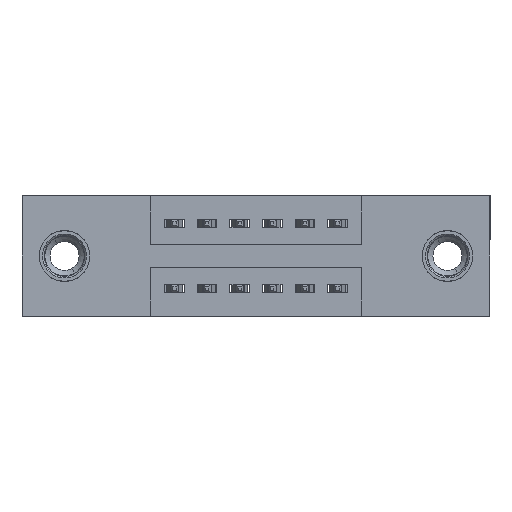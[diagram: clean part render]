
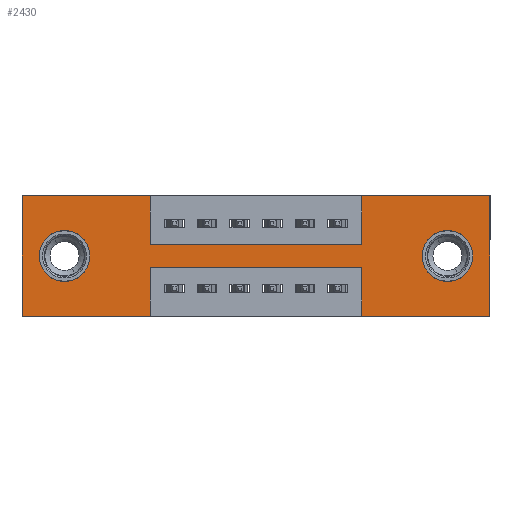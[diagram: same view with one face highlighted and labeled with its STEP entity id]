
A CAD part, front view. The second image highlights one B-rep face of the part: STEP entity #2430.
In plain terms, the highlighted planar face has unit normal (0, -1, 0).
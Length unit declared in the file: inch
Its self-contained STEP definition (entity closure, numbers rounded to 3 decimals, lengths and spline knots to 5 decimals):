
#135 = VECTOR ( 'NONE', #530, 39.37008 ) ;
#219 = CARTESIAN_POINT ( 'NONE',  ( 1.0425, 0., -0.37 ) ) ;
#243 = VERTEX_POINT ( 'NONE', #446 ) ;
#343 = CARTESIAN_POINT ( 'NONE',  ( 0., 0., -0.37 ) ) ;
#446 = CARTESIAN_POINT ( 'NONE',  ( 1.435, 0., -0.37 ) ) ;
#457 = AXIS2_PLACEMENT_3D ( 'NONE', #11871, #5175, #12933 ) ;
#530 = DIRECTION ( 'NONE',  ( 0., 0., -1. ) ) ;
#587 = EDGE_CURVE ( 'NONE', #9913, #12338, #13255, .T. ) ;
#811 = EDGE_CURVE ( 'NONE', #7252, #1962, #5625, .T. ) ;
#879 = CIRCLE ( 'NONE', #991, 0.078 ) ;
#899 = ORIENTED_EDGE ( 'NONE', *, *, #9213, .F. ) ;
#991 = AXIS2_PLACEMENT_3D ( 'NONE', #6769, #6752, #6735 ) ;
#1046 = DIRECTION ( 'NONE',  ( 0., 1., 0. ) ) ;
#1078 = CARTESIAN_POINT ( 'NONE',  ( 1.305, 0., -0.185 ) ) ;
#1255 = EDGE_CURVE ( 'NONE', #6363, #8230, #2990, .T. ) ;
#1276 = VERTEX_POINT ( 'NONE', #3013 ) ;
#1614 = ORIENTED_EDGE ( 'NONE', *, *, #587, .F. ) ;
#1720 = CIRCLE ( 'NONE', #8643, 0.078 ) ;
#1917 = EDGE_CURVE ( 'NONE', #8348, #11633, #879, .T. ) ;
#1962 = VERTEX_POINT ( 'NONE', #4195 ) ;
#2200 = DIRECTION ( 'NONE',  ( 0., 0., -1. ) ) ;
#2403 = CIRCLE ( 'NONE', #13625, 0.078 ) ;
#2430 = ADVANCED_FACE ( 'NONE', ( #9476, #6102, #3129 ), #8458, .T. ) ;
#2528 = DIRECTION ( 'NONE',  ( 0., 0., -1. ) ) ;
#2545 = CARTESIAN_POINT ( 'NONE',  ( 0.3925, 0., -0.37 ) ) ;
#2904 = DIRECTION ( 'NONE',  ( -1., 0., 0. ) ) ;
#2976 = ORIENTED_EDGE ( 'NONE', *, *, #5155, .T. ) ;
#2990 = LINE ( 'NONE', #3721, #5611 ) ;
#3013 = CARTESIAN_POINT ( 'NONE',  ( 0.13, 0., -0.263 ) ) ;
#3057 = VECTOR ( 'NONE', #3636, 39.37008 ) ;
#3074 = CARTESIAN_POINT ( 'NONE',  ( 0.3925, 0., -0.22 ) ) ;
#3129 = FACE_OUTER_BOUND ( 'NONE', #7945, .T. ) ;
#3355 = CARTESIAN_POINT ( 'NONE',  ( 1.0425, 0., -0.15 ) ) ;
#3531 = DIRECTION ( 'NONE',  ( 1., 0., 0. ) ) ;
#3549 = EDGE_CURVE ( 'NONE', #8230, #6607, #10190, .T. ) ;
#3564 = EDGE_LOOP ( 'NONE', ( #2976, #11907 ) ) ;
#3636 = DIRECTION ( 'NONE',  ( 0., 0., -1. ) ) ;
#3654 = DIRECTION ( 'NONE',  ( 1., 0., 0. ) ) ;
#3661 = ORIENTED_EDGE ( 'NONE', *, *, #14028, .F. ) ;
#3677 = DIRECTION ( 'NONE',  ( -1., 0., 0. ) ) ;
#3721 = CARTESIAN_POINT ( 'NONE',  ( 0.3925, 0., -0.22 ) ) ;
#4195 = CARTESIAN_POINT ( 'NONE',  ( 1.0425, 0., 0. ) ) ;
#4563 = CARTESIAN_POINT ( 'NONE',  ( 0.3925, 0., 0. ) ) ;
#4630 = VECTOR ( 'NONE', #3531, 39.37008 ) ;
#4744 = EDGE_CURVE ( 'NONE', #1276, #12189, #2403, .T. ) ;
#4755 = CARTESIAN_POINT ( 'NONE',  ( 1.0425, 0., -0.37 ) ) ;
#4912 = LINE ( 'NONE', #10435, #13706 ) ;
#5014 = CARTESIAN_POINT ( 'NONE',  ( 1.435, 0., 0. ) ) ;
#5155 = EDGE_CURVE ( 'NONE', #12189, #1276, #9013, .T. ) ;
#5175 = DIRECTION ( 'NONE',  ( 0., 1., 0. ) ) ;
#5250 = ORIENTED_EDGE ( 'NONE', *, *, #8855, .T. ) ;
#5261 = EDGE_LOOP ( 'NONE', ( #5250, #14034 ) ) ;
#5561 = EDGE_CURVE ( 'NONE', #243, #9596, #12590, .T. ) ;
#5611 = VECTOR ( 'NONE', #2904, 39.37008 ) ;
#5625 = LINE ( 'NONE', #10940, #7953 ) ;
#5860 = DIRECTION ( 'NONE',  ( 0., 0., 1. ) ) ;
#6029 = LINE ( 'NONE', #7006, #3057 ) ;
#6042 = VECTOR ( 'NONE', #8165, 39.37008 ) ;
#6102 = FACE_BOUND ( 'NONE', #3564, .T. ) ;
#6363 = VERTEX_POINT ( 'NONE', #10796 ) ;
#6518 = CARTESIAN_POINT ( 'NONE',  ( 0.13, 0., -0.107 ) ) ;
#6558 = CARTESIAN_POINT ( 'NONE',  ( 1.305, 0., -0.263 ) ) ;
#6607 = VERTEX_POINT ( 'NONE', #8963 ) ;
#6735 = DIRECTION ( 'NONE',  ( 0., 0., -1. ) ) ;
#6752 = DIRECTION ( 'NONE',  ( 0., 1., 0. ) ) ;
#6769 = CARTESIAN_POINT ( 'NONE',  ( 1.305, 0., -0.185 ) ) ;
#6955 = VERTEX_POINT ( 'NONE', #11870 ) ;
#7006 = CARTESIAN_POINT ( 'NONE',  ( 1.435, 0., 0. ) ) ;
#7252 = VERTEX_POINT ( 'NONE', #3355 ) ;
#7458 = CARTESIAN_POINT ( 'NONE',  ( 0., 0., 0. ) ) ;
#7752 = ORIENTED_EDGE ( 'NONE', *, *, #10187, .F. ) ;
#7776 = CARTESIAN_POINT ( 'NONE',  ( 0.13, 0., -0.185 ) ) ;
#7945 = EDGE_LOOP ( 'NONE', ( #9326, #12249, #3661, #12889, #7752, #13873, #11400, #9169, #899, #1614, #8289, #11576 ) ) ;
#7953 = VECTOR ( 'NONE', #9602, 39.37008 ) ;
#8165 = DIRECTION ( 'NONE',  ( 0., 0., 1. ) ) ;
#8230 = VERTEX_POINT ( 'NONE', #3074 ) ;
#8269 = DIRECTION ( 'NONE',  ( 0., 0., -1. ) ) ;
#8289 = ORIENTED_EDGE ( 'NONE', *, *, #9682, .F. ) ;
#8337 = EDGE_CURVE ( 'NONE', #6607, #6955, #12849, .T. ) ;
#8348 = VERTEX_POINT ( 'NONE', #6558 ) ;
#8370 = DIRECTION ( 'NONE',  ( 0., -1., 0. ) ) ;
#8407 = CARTESIAN_POINT ( 'NONE',  ( 0.3925, 0., -0.15 ) ) ;
#8458 = PLANE ( 'NONE',  #11943 ) ;
#8643 = AXIS2_PLACEMENT_3D ( 'NONE', #1078, #8946, #2200 ) ;
#8773 = CARTESIAN_POINT ( 'NONE',  ( 0., 0., -0.37 ) ) ;
#8855 = EDGE_CURVE ( 'NONE', #11633, #8348, #1720, .T. ) ;
#8915 = DIRECTION ( 'NONE',  ( 0., 0., 1. ) ) ;
#8946 = DIRECTION ( 'NONE',  ( 0., 1., 0. ) ) ;
#8963 = CARTESIAN_POINT ( 'NONE',  ( 0.3925, 0., -0.37 ) ) ;
#9013 = CIRCLE ( 'NONE', #457, 0.078 ) ;
#9169 = ORIENTED_EDGE ( 'NONE', *, *, #10774, .F. ) ;
#9213 = EDGE_CURVE ( 'NONE', #12338, #12538, #12013, .T. ) ;
#9321 = DIRECTION ( 'NONE',  ( 1., 0., 0. ) ) ;
#9326 = ORIENTED_EDGE ( 'NONE', *, *, #3549, .F. ) ;
#9476 = FACE_BOUND ( 'NONE', #5261, .T. ) ;
#9596 = VERTEX_POINT ( 'NONE', #219 ) ;
#9602 = DIRECTION ( 'NONE',  ( 0., 0., 1. ) ) ;
#9682 = EDGE_CURVE ( 'NONE', #6955, #9913, #12003, .T. ) ;
#9692 = VECTOR ( 'NONE', #3677, 39.37008 ) ;
#9828 = VECTOR ( 'NONE', #2528, 39.37008 ) ;
#9913 = VERTEX_POINT ( 'NONE', #7458 ) ;
#9935 = CARTESIAN_POINT ( 'NONE',  ( 0., 0., -0.37 ) ) ;
#9999 = VECTOR ( 'NONE', #13167, 39.37008 ) ;
#10187 = EDGE_CURVE ( 'NONE', #13062, #243, #6029, .T. ) ;
#10190 = LINE ( 'NONE', #2545, #9828 ) ;
#10418 = VECTOR ( 'NONE', #9321, 39.37008 ) ;
#10435 = CARTESIAN_POINT ( 'NONE',  ( 0., 0., 0. ) ) ;
#10616 = LINE ( 'NONE', #11339, #4630 ) ;
#10774 = EDGE_CURVE ( 'NONE', #12538, #7252, #10616, .T. ) ;
#10796 = CARTESIAN_POINT ( 'NONE',  ( 1.0425, 0., -0.22 ) ) ;
#10940 = CARTESIAN_POINT ( 'NONE',  ( 1.0425, 0., 0. ) ) ;
#11339 = CARTESIAN_POINT ( 'NONE',  ( 0.3925, 0., -0.15 ) ) ;
#11400 = ORIENTED_EDGE ( 'NONE', *, *, #811, .F. ) ;
#11567 = VECTOR ( 'NONE', #5860, 39.37008 ) ;
#11576 = ORIENTED_EDGE ( 'NONE', *, *, #8337, .F. ) ;
#11633 = VERTEX_POINT ( 'NONE', #14129 ) ;
#11870 = CARTESIAN_POINT ( 'NONE',  ( 0., 0., -0.37 ) ) ;
#11871 = CARTESIAN_POINT ( 'NONE',  ( 0.13, 0., -0.185 ) ) ;
#11891 = CARTESIAN_POINT ( 'NONE',  ( 0., 0., 0. ) ) ;
#11907 = ORIENTED_EDGE ( 'NONE', *, *, #4744, .T. ) ;
#11943 = AXIS2_PLACEMENT_3D ( 'NONE', #8773, #8370, #8269 ) ;
#12003 = LINE ( 'NONE', #13629, #6042 ) ;
#12013 = LINE ( 'NONE', #13783, #135 ) ;
#12189 = VERTEX_POINT ( 'NONE', #6518 ) ;
#12249 = ORIENTED_EDGE ( 'NONE', *, *, #1255, .F. ) ;
#12338 = VERTEX_POINT ( 'NONE', #4563 ) ;
#12538 = VERTEX_POINT ( 'NONE', #8407 ) ;
#12590 = LINE ( 'NONE', #343, #9692 ) ;
#12849 = LINE ( 'NONE', #9935, #9999 ) ;
#12889 = ORIENTED_EDGE ( 'NONE', *, *, #5561, .F. ) ;
#12933 = DIRECTION ( 'NONE',  ( 0., 0., 1. ) ) ;
#13062 = VERTEX_POINT ( 'NONE', #5014 ) ;
#13167 = DIRECTION ( 'NONE',  ( -1., 0., 0. ) ) ;
#13255 = LINE ( 'NONE', #11891, #10418 ) ;
#13625 = AXIS2_PLACEMENT_3D ( 'NONE', #7776, #1046, #8915 ) ;
#13629 = CARTESIAN_POINT ( 'NONE',  ( 0., 0., 0. ) ) ;
#13706 = VECTOR ( 'NONE', #3654, 39.37008 ) ;
#13783 = CARTESIAN_POINT ( 'NONE',  ( 0.3925, 0., 0. ) ) ;
#13873 = ORIENTED_EDGE ( 'NONE', *, *, #14047, .F. ) ;
#14028 = EDGE_CURVE ( 'NONE', #9596, #6363, #14035, .T. ) ;
#14034 = ORIENTED_EDGE ( 'NONE', *, *, #1917, .T. ) ;
#14035 = LINE ( 'NONE', #4755, #11567 ) ;
#14047 = EDGE_CURVE ( 'NONE', #1962, #13062, #4912, .T. ) ;
#14129 = CARTESIAN_POINT ( 'NONE',  ( 1.305, 0., -0.107 ) ) ;
